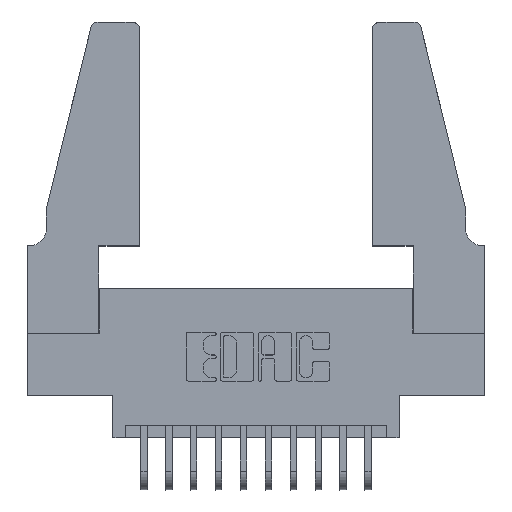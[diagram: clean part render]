
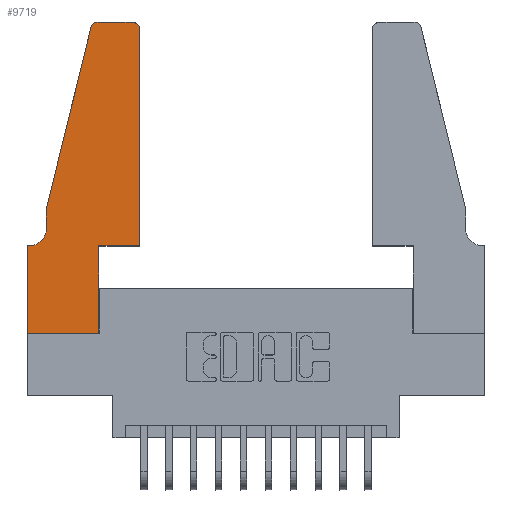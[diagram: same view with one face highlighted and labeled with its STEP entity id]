
A CAD part, top view. The second image highlights one B-rep face of the part: STEP entity #9719.
In plain terms, the highlighted planar face has unit normal (0, 0, 1).
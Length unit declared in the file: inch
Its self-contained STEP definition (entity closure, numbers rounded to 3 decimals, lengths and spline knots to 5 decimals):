
#492 = CARTESIAN_POINT ( 'NONE',  ( 0.25487, 1.22718, 0.37 ) ) ;
#789 = DIRECTION ( 'NONE',  ( -1., 0., 0. ) ) ;
#829 = EDGE_CURVE ( 'NONE', #3585, #5875, #1933, .T. ) ;
#878 = EDGE_CURVE ( 'NONE', #12544, #3585, #4464, .T. ) ;
#1433 = CARTESIAN_POINT ( 'NONE',  ( 0.0755, 0.5, 0.37 ) ) ;
#1678 = CARTESIAN_POINT ( 'NONE',  ( 0.284, 1.25, 0.37 ) ) ;
#1831 = DIRECTION ( 'NONE',  ( 0., 0., 1. ) ) ;
#1933 = LINE ( 'NONE', #10481, #11462 ) ;
#2433 = VERTEX_POINT ( 'NONE', #11725 ) ;
#2613 = LINE ( 'NONE', #15368, #15396 ) ;
#2769 = VECTOR ( 'NONE', #7633, 39.37008 ) ;
#2897 = ORIENTED_EDGE ( 'NONE', *, *, #878, .T. ) ;
#2931 = EDGE_CURVE ( 'NONE', #5220, #13355, #10679, .T. ) ;
#2964 = FACE_OUTER_BOUND ( 'NONE', #10094, .T. ) ;
#3420 = AXIS2_PLACEMENT_3D ( 'NONE', #14586, #12174, #4759 ) ;
#3506 = ORIENTED_EDGE ( 'NONE', *, *, #7179, .T. ) ;
#3585 = VERTEX_POINT ( 'NONE', #5795 ) ;
#3586 = DIRECTION ( 'NONE',  ( -1., 0., 0. ) ) ;
#3604 = EDGE_CURVE ( 'NONE', #13355, #10565, #13692, .T. ) ;
#3650 = VERTEX_POINT ( 'NONE', #492 ) ;
#3680 = VERTEX_POINT ( 'NONE', #8362 ) ;
#4014 = LINE ( 'NONE', #1433, #10677 ) ;
#4384 = CARTESIAN_POINT ( 'NONE',  ( 0.0755, 0.42, 0.37 ) ) ;
#4402 = DIRECTION ( 'NONE',  ( 0., -1., 0. ) ) ;
#4464 = LINE ( 'NONE', #15231, #14330 ) ;
#4759 = DIRECTION ( 'NONE',  ( 1., 0., 0. ) ) ;
#4845 = EDGE_CURVE ( 'NONE', #8913, #5220, #10244, .T. ) ;
#5220 = VERTEX_POINT ( 'NONE', #6442 ) ;
#5312 = AXIS2_PLACEMENT_3D ( 'NONE', #9320, #1831, #10571 ) ;
#5514 = CARTESIAN_POINT ( 'NONE',  ( 0.4505, 0.35, 0.37 ) ) ;
#5617 = CIRCLE ( 'NONE', #5312, 0.03 ) ;
#5795 = CARTESIAN_POINT ( 'NONE',  ( 0.2865, 0.35, 0.37 ) ) ;
#5824 = EDGE_CURVE ( 'NONE', #3650, #2433, #9828, .T. ) ;
#5875 = VERTEX_POINT ( 'NONE', #7680 ) ;
#6185 = DIRECTION ( 'NONE',  ( 0., 0., 1. ) ) ;
#6442 = CARTESIAN_POINT ( 'NONE',  ( 0.0055, 0.35, 0.37 ) ) ;
#6586 = ORIENTED_EDGE ( 'NONE', *, *, #2931, .T. ) ;
#6751 = EDGE_CURVE ( 'NONE', #5875, #3680, #7011, .T. ) ;
#6785 = DIRECTION ( 'NONE',  ( 0., 1., 0. ) ) ;
#7011 = LINE ( 'NONE', #5514, #13150 ) ;
#7179 = EDGE_CURVE ( 'NONE', #2433, #8913, #4014, .T. ) ;
#7236 = PLANE ( 'NONE',  #3420 ) ;
#7280 = CARTESIAN_POINT ( 'NONE',  ( 0.0755, 0.35, 0.37 ) ) ;
#7396 = VECTOR ( 'NONE', #3586, 39.37008 ) ;
#7633 = DIRECTION ( 'NONE',  ( -0.239, -0.971, 0. ) ) ;
#7680 = CARTESIAN_POINT ( 'NONE',  ( 0.4505, 0.35, 0.37 ) ) ;
#7695 = DIRECTION ( 'NONE',  ( 0., -1., 0. ) ) ;
#7966 = ORIENTED_EDGE ( 'NONE', *, *, #10576, .T. ) ;
#8183 = CARTESIAN_POINT ( 'NONE',  ( 0.2605, 1.25, 0.37 ) ) ;
#8221 = AXIS2_PLACEMENT_3D ( 'NONE', #15646, #8298, #789 ) ;
#8298 = DIRECTION ( 'NONE',  ( 0., 0., -1. ) ) ;
#8362 = CARTESIAN_POINT ( 'NONE',  ( 0.4505, 1.22, 0.37 ) ) ;
#8527 = ORIENTED_EDGE ( 'NONE', *, *, #6751, .T. ) ;
#8844 = EDGE_CURVE ( 'NONE', #10565, #12544, #2613, .T. ) ;
#8913 = VERTEX_POINT ( 'NONE', #4384 ) ;
#9044 = ORIENTED_EDGE ( 'NONE', *, *, #8844, .T. ) ;
#9079 = CARTESIAN_POINT ( 'NONE',  ( 0., 0.35, 0.37 ) ) ;
#9082 = ORIENTED_EDGE ( 'NONE', *, *, #5824, .T. ) ;
#9265 = DIRECTION ( 'NONE',  ( 1., 0., 0. ) ) ;
#9320 = CARTESIAN_POINT ( 'NONE',  ( 0.4205, 1.22, 0.37 ) ) ;
#9424 = DIRECTION ( 'NONE',  ( -1., 0., 0. ) ) ;
#9576 = ORIENTED_EDGE ( 'NONE', *, *, #4845, .T. ) ;
#9719 = ADVANCED_FACE ( 'NONE', ( #2964 ), #7236, .T. ) ;
#9828 = LINE ( 'NONE', #12501, #2769 ) ;
#10094 = EDGE_LOOP ( 'NONE', ( #7966, #10746, #9082, #3506, #9576, #6586, #10790, #9044, #2897, #14836, #8527, #14180 ) ) ;
#10244 = CIRCLE ( 'NONE', #8221, 0.07 ) ;
#10310 = CIRCLE ( 'NONE', #11704, 0.03 ) ;
#10466 = VECTOR ( 'NONE', #4402, 39.37008 ) ;
#10481 = CARTESIAN_POINT ( 'NONE',  ( 0.4505, 0.35, 0.37 ) ) ;
#10565 = VERTEX_POINT ( 'NONE', #14277 ) ;
#10571 = DIRECTION ( 'NONE',  ( 1., 0., 0. ) ) ;
#10576 = EDGE_CURVE ( 'NONE', #11764, #11565, #10761, .T. ) ;
#10677 = VECTOR ( 'NONE', #7695, 39.37008 ) ;
#10679 = LINE ( 'NONE', #7280, #7396 ) ;
#10746 = ORIENTED_EDGE ( 'NONE', *, *, #15603, .T. ) ;
#10761 = LINE ( 'NONE', #8183, #13214 ) ;
#10790 = ORIENTED_EDGE ( 'NONE', *, *, #3604, .T. ) ;
#10855 = CARTESIAN_POINT ( 'NONE',  ( 0.4205, 1.25, 0.37 ) ) ;
#11462 = VECTOR ( 'NONE', #14734, 39.37008 ) ;
#11565 = VERTEX_POINT ( 'NONE', #1678 ) ;
#11704 = AXIS2_PLACEMENT_3D ( 'NONE', #13554, #6185, #14791 ) ;
#11725 = CARTESIAN_POINT ( 'NONE',  ( 0.0755, 0.5, 0.37 ) ) ;
#11764 = VERTEX_POINT ( 'NONE', #10855 ) ;
#12174 = DIRECTION ( 'NONE',  ( 0., 0., 1. ) ) ;
#12304 = CARTESIAN_POINT ( 'NONE',  ( 0.2865, 0., 0.37 ) ) ;
#12501 = CARTESIAN_POINT ( 'NONE',  ( 0.0755, 0.5, 0.37 ) ) ;
#12544 = VERTEX_POINT ( 'NONE', #12304 ) ;
#13150 = VECTOR ( 'NONE', #6785, 39.37008 ) ;
#13214 = VECTOR ( 'NONE', #9424, 39.37008 ) ;
#13355 = VERTEX_POINT ( 'NONE', #9079 ) ;
#13554 = CARTESIAN_POINT ( 'NONE',  ( 0.284, 1.22, 0.37 ) ) ;
#13692 = LINE ( 'NONE', #15576, #10466 ) ;
#14180 = ORIENTED_EDGE ( 'NONE', *, *, #15920, .T. ) ;
#14277 = CARTESIAN_POINT ( 'NONE',  ( 0., 0., 0.37 ) ) ;
#14330 = VECTOR ( 'NONE', #14546, 39.37008 ) ;
#14546 = DIRECTION ( 'NONE',  ( 0., 1., 0. ) ) ;
#14586 = CARTESIAN_POINT ( 'NONE',  ( 0., 0.35, 0.37 ) ) ;
#14734 = DIRECTION ( 'NONE',  ( 1., 0., 0. ) ) ;
#14791 = DIRECTION ( 'NONE',  ( 1., 0., 0. ) ) ;
#14836 = ORIENTED_EDGE ( 'NONE', *, *, #829, .T. ) ;
#15231 = CARTESIAN_POINT ( 'NONE',  ( 0.2865, 0.35, 0.37 ) ) ;
#15368 = CARTESIAN_POINT ( 'NONE',  ( 0., 0., 0.37 ) ) ;
#15396 = VECTOR ( 'NONE', #9265, 39.37008 ) ;
#15576 = CARTESIAN_POINT ( 'NONE',  ( 0., 0., 0.37 ) ) ;
#15603 = EDGE_CURVE ( 'NONE', #11565, #3650, #10310, .T. ) ;
#15646 = CARTESIAN_POINT ( 'NONE',  ( 0.0055, 0.42, 0.37 ) ) ;
#15920 = EDGE_CURVE ( 'NONE', #3680, #11764, #5617, .T. ) ;
